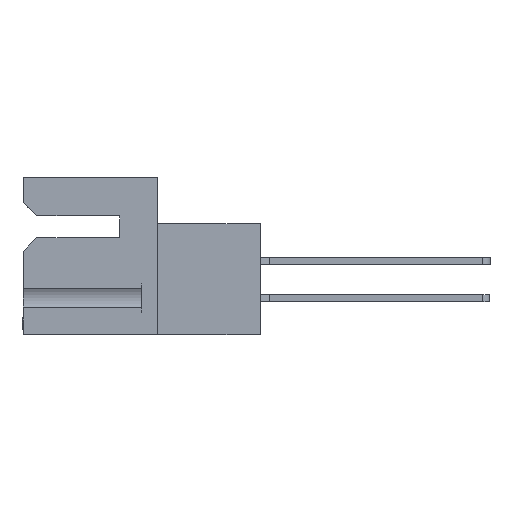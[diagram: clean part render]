
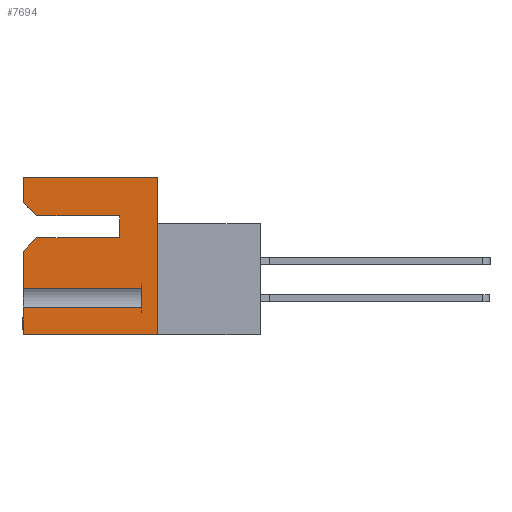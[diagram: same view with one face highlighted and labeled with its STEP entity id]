
A CAD part, left-side view. The second image highlights one B-rep face of the part: STEP entity #7694.
In plain terms, the highlighted planar face has unit normal (-1, 0, 0).
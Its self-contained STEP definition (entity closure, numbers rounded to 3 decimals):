
#77 = EDGE_CURVE ( 'NONE', #28235, #32586, #5315, .T. ) ;
#517 = VERTEX_POINT ( 'NONE', #3155 ) ;
#630 = CARTESIAN_POINT ( 'NONE',  ( 0., 11.506, 0. ) ) ;
#1701 = CARTESIAN_POINT ( 'NONE',  ( 0., 11.506, -13.487 ) ) ;
#1903 = ORIENTED_EDGE ( 'NONE', *, *, #15967, .F. ) ;
#1958 = DIRECTION ( 'NONE',  ( 0., 0.707, -0.707 ) ) ;
#2639 = CARTESIAN_POINT ( 'NONE',  ( 0., 10.363, -3.302 ) ) ;
#3078 = EDGE_LOOP ( 'NONE', ( #1903, #18436, #3119, #36888, #20502, #35457, #27992, #7066, #17121, #11669, #25580, #11862, #28609, #15877 ) ) ;
#3119 = ORIENTED_EDGE ( 'NONE', *, *, #34961, .F. ) ;
#3155 = CARTESIAN_POINT ( 'NONE',  ( 0., 3.251, -5.182 ) ) ;
#3582 = VECTOR ( 'NONE', #20907, 1000. ) ;
#4016 = EDGE_CURVE ( 'NONE', #31786, #26348, #13170, .T. ) ;
#5315 = LINE ( 'NONE', #21581, #12506 ) ;
#6523 = VECTOR ( 'NONE', #18788, 1000. ) ;
#6779 = VECTOR ( 'NONE', #43502, 1000. ) ;
#7066 = ORIENTED_EDGE ( 'NONE', *, *, #32910, .F. ) ;
#7647 = VECTOR ( 'NONE', #32374, 1000. ) ;
#7694 = ADVANCED_FACE ( 'NONE', ( #44644 ), #14136, .F. ) ;
#8144 = EDGE_CURVE ( 'NONE', #22197, #8923, #31305, .T. ) ;
#8483 = CARTESIAN_POINT ( 'NONE',  ( 0., 11.506, -9.556 ) ) ;
#8871 = LINE ( 'NONE', #20355, #21626 ) ;
#8923 = VERTEX_POINT ( 'NONE', #16259 ) ;
#10057 = LINE ( 'NONE', #26224, #45509 ) ;
#10869 = DIRECTION ( 'NONE',  ( 1., 0., 0. ) ) ;
#11008 = VERTEX_POINT ( 'NONE', #44790 ) ;
#11669 = ORIENTED_EDGE ( 'NONE', *, *, #4016, .F. ) ;
#11862 = ORIENTED_EDGE ( 'NONE', *, *, #12240, .F. ) ;
#12240 = EDGE_CURVE ( 'NONE', #28235, #20674, #41081, .T. ) ;
#12506 = VECTOR ( 'NONE', #28383, 1000. ) ;
#12760 = DIRECTION ( 'NONE',  ( 0., 0., 1. ) ) ;
#13070 = VECTOR ( 'NONE', #36959, 1000. ) ;
#13170 = LINE ( 'NONE', #45472, #25374 ) ;
#13737 = DIRECTION ( 'NONE',  ( 0., 0., 1. ) ) ;
#14136 = PLANE ( 'NONE',  #45372 ) ;
#14719 = EDGE_CURVE ( 'NONE', #517, #31355, #41739, .T. ) ;
#15877 = ORIENTED_EDGE ( 'NONE', *, *, #17454, .F. ) ;
#15937 = LINE ( 'NONE', #1701, #6523 ) ;
#15967 = EDGE_CURVE ( 'NONE', #8923, #11008, #22751, .T. ) ;
#16259 = CARTESIAN_POINT ( 'NONE',  ( 0., 0., -13.487 ) ) ;
#16367 = CARTESIAN_POINT ( 'NONE',  ( 0., 1.346, -11.17 ) ) ;
#17021 = CARTESIAN_POINT ( 'NONE',  ( 0., 0., 0. ) ) ;
#17102 = LINE ( 'NONE', #45631, #40419 ) ;
#17121 = ORIENTED_EDGE ( 'NONE', *, *, #29816, .T. ) ;
#17454 = EDGE_CURVE ( 'NONE', #11008, #32586, #8871, .T. ) ;
#17471 = CARTESIAN_POINT ( 'NONE',  ( 0., 0., 0. ) ) ;
#17598 = CARTESIAN_POINT ( 'NONE',  ( 0., 1.346, 0. ) ) ;
#17818 = CARTESIAN_POINT ( 'NONE',  ( 0., 0., -3.302 ) ) ;
#18436 = ORIENTED_EDGE ( 'NONE', *, *, #8144, .F. ) ;
#18788 = DIRECTION ( 'NONE',  ( 0., 0., 1. ) ) ;
#20355 = CARTESIAN_POINT ( 'NONE',  ( 0., 11.506, -13.487 ) ) ;
#20502 = ORIENTED_EDGE ( 'NONE', *, *, #39564, .T. ) ;
#20674 = VERTEX_POINT ( 'NONE', #27007 ) ;
#20907 = DIRECTION ( 'NONE',  ( 0., 0., -1. ) ) ;
#21581 = CARTESIAN_POINT ( 'NONE',  ( 0., 1.346, -11.17 ) ) ;
#21626 = VECTOR ( 'NONE', #12760, 1000. ) ;
#22141 = CARTESIAN_POINT ( 'NONE',  ( 0., 3.251, -5.182 ) ) ;
#22197 = VERTEX_POINT ( 'NONE', #17021 ) ;
#22751 = LINE ( 'NONE', #38911, #45499 ) ;
#23636 = DIRECTION ( 'NONE',  ( 0., 0., 1. ) ) ;
#24532 = CARTESIAN_POINT ( 'NONE',  ( 0., 10.363, -3.302 ) ) ;
#24674 = DIRECTION ( 'NONE',  ( 0., -0.707, -0.707 ) ) ;
#24951 = CARTESIAN_POINT ( 'NONE',  ( 0., 11.506, -2.159 ) ) ;
#25374 = VECTOR ( 'NONE', #23636, 1000. ) ;
#25402 = DIRECTION ( 'NONE',  ( 0., 1., 0. ) ) ;
#25446 = EDGE_CURVE ( 'NONE', #31355, #29327, #39817, .T. ) ;
#25580 = ORIENTED_EDGE ( 'NONE', *, *, #27197, .T. ) ;
#25688 = VECTOR ( 'NONE', #24674, 1000. ) ;
#25926 = LINE ( 'NONE', #34073, #36480 ) ;
#26224 = CARTESIAN_POINT ( 'NONE',  ( 0., 11.506, 0. ) ) ;
#26348 = VERTEX_POINT ( 'NONE', #43405 ) ;
#27007 = CARTESIAN_POINT ( 'NONE',  ( 0., 1.346, -9.556 ) ) ;
#27197 = EDGE_CURVE ( 'NONE', #31786, #20674, #36883, .T. ) ;
#27904 = CARTESIAN_POINT ( 'NONE',  ( 0., 10.363, -5.182 ) ) ;
#27992 = ORIENTED_EDGE ( 'NONE', *, *, #14719, .F. ) ;
#28235 = VERTEX_POINT ( 'NONE', #16367 ) ;
#28307 = VECTOR ( 'NONE', #13737, 1000. ) ;
#28383 = DIRECTION ( 'NONE',  ( 0., 1., 0. ) ) ;
#28609 = ORIENTED_EDGE ( 'NONE', *, *, #77, .T. ) ;
#29327 = VERTEX_POINT ( 'NONE', #2639 ) ;
#29811 = CARTESIAN_POINT ( 'NONE',  ( 0., 1.346, -9.556 ) ) ;
#29816 = EDGE_CURVE ( 'NONE', #40091, #26348, #25926, .T. ) ;
#31305 = LINE ( 'NONE', #17471, #3582 ) ;
#31355 = VERTEX_POINT ( 'NONE', #36445 ) ;
#31786 = VERTEX_POINT ( 'NONE', #8483 ) ;
#32374 = DIRECTION ( 'NONE',  ( 0., 1., 0. ) ) ;
#32586 = VERTEX_POINT ( 'NONE', #44260 ) ;
#32910 = EDGE_CURVE ( 'NONE', #40091, #517, #17102, .T. ) ;
#33854 = EDGE_CURVE ( 'NONE', #41292, #45704, #15937, .T. ) ;
#34073 = CARTESIAN_POINT ( 'NONE',  ( 0., 10.363, -5.182 ) ) ;
#34961 = EDGE_CURVE ( 'NONE', #45704, #22197, #10057, .T. ) ;
#35457 = ORIENTED_EDGE ( 'NONE', *, *, #25446, .F. ) ;
#36445 = CARTESIAN_POINT ( 'NONE',  ( 0., 3.251, -3.302 ) ) ;
#36480 = VECTOR ( 'NONE', #1958, 1000. ) ;
#36883 = LINE ( 'NONE', #29811, #13070 ) ;
#36888 = ORIENTED_EDGE ( 'NONE', *, *, #33854, .F. ) ;
#36959 = DIRECTION ( 'NONE',  ( 0., -1., 0. ) ) ;
#38911 = CARTESIAN_POINT ( 'NONE',  ( 0., -8.814, -13.487 ) ) ;
#38986 = DIRECTION ( 'NONE',  ( 0., -1., 0. ) ) ;
#39564 = EDGE_CURVE ( 'NONE', #41292, #29327, #43418, .T. ) ;
#39817 = LINE ( 'NONE', #17818, #7647 ) ;
#40091 = VERTEX_POINT ( 'NONE', #27904 ) ;
#40419 = VECTOR ( 'NONE', #38986, 1000. ) ;
#41081 = LINE ( 'NONE', #17598, #28307 ) ;
#41292 = VERTEX_POINT ( 'NONE', #24951 ) ;
#41739 = LINE ( 'NONE', #22141, #6779 ) ;
#42952 = CARTESIAN_POINT ( 'NONE',  ( 0., 0., 0. ) ) ;
#43105 = DIRECTION ( 'NONE',  ( 0., 0., -1. ) ) ;
#43405 = CARTESIAN_POINT ( 'NONE',  ( 0., 11.506, -6.325 ) ) ;
#43418 = LINE ( 'NONE', #24532, #25688 ) ;
#43502 = DIRECTION ( 'NONE',  ( 0., 0., 1. ) ) ;
#44160 = DIRECTION ( 'NONE',  ( 0., -1., 0. ) ) ;
#44260 = CARTESIAN_POINT ( 'NONE',  ( 0., 11.506, -11.17 ) ) ;
#44644 = FACE_OUTER_BOUND ( 'NONE', #3078, .T. ) ;
#44790 = CARTESIAN_POINT ( 'NONE',  ( 0., 11.506, -13.487 ) ) ;
#45372 = AXIS2_PLACEMENT_3D ( 'NONE', #42952, #10869, #43105 ) ;
#45472 = CARTESIAN_POINT ( 'NONE',  ( 0., 11.506, -13.487 ) ) ;
#45499 = VECTOR ( 'NONE', #25402, 1000. ) ;
#45509 = VECTOR ( 'NONE', #44160, 1000. ) ;
#45631 = CARTESIAN_POINT ( 'NONE',  ( 0., 0., -5.182 ) ) ;
#45704 = VERTEX_POINT ( 'NONE', #630 ) ;
